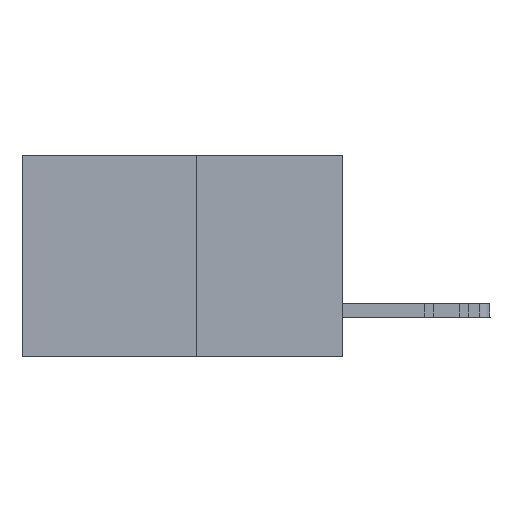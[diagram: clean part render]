
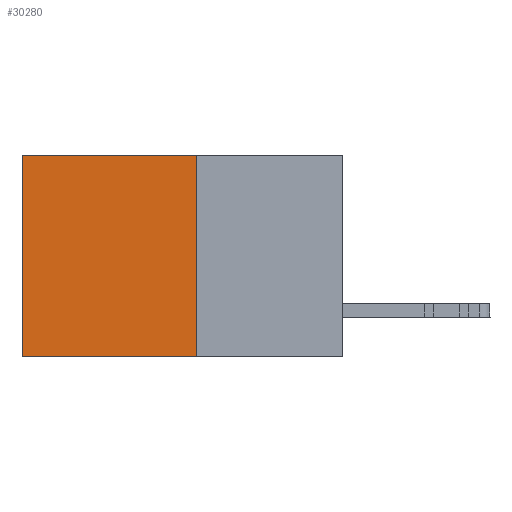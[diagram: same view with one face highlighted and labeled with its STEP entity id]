
A CAD part, left-side view. The second image highlights one B-rep face of the part: STEP entity #30280.
In plain terms, the highlighted planar face has unit normal (-1, 0, 0).
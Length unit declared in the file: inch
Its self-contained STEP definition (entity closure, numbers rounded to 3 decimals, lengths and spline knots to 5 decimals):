
#276 = VERTEX_POINT ( 'NONE', #27591 ) ;
#533 = LINE ( 'NONE', #15599, #6340 ) ;
#884 = ORIENTED_EDGE ( 'NONE', *, *, #6811, .T. ) ;
#2942 = FACE_OUTER_BOUND ( 'NONE', #16641, .T. ) ;
#3382 = DIRECTION ( 'NONE',  ( 0., 0., -1. ) ) ;
#3504 = ORIENTED_EDGE ( 'NONE', *, *, #21142, .T. ) ;
#3750 = LINE ( 'NONE', #5084, #10233 ) ;
#4756 = VERTEX_POINT ( 'NONE', #24089 ) ;
#5084 = CARTESIAN_POINT ( 'NONE',  ( 0.277, 0.27, -0.37 ) ) ;
#6340 = VECTOR ( 'NONE', #3382, 39.37008 ) ;
#6811 = EDGE_CURVE ( 'NONE', #13426, #9421, #27106, .T. ) ;
#7402 = PLANE ( 'NONE',  #9200 ) ;
#7548 = DIRECTION ( 'NONE',  ( 0., 1., 0. ) ) ;
#9200 = AXIS2_PLACEMENT_3D ( 'NONE', #23743, #9836, #27063 ) ;
#9295 = DIRECTION ( 'NONE',  ( 0., 0., -1. ) ) ;
#9328 = CARTESIAN_POINT ( 'NONE',  ( 0.277, 0.59, -0.37 ) ) ;
#9421 = VERTEX_POINT ( 'NONE', #14662 ) ;
#9836 = DIRECTION ( 'NONE',  ( 1., 0., 0. ) ) ;
#10233 = VECTOR ( 'NONE', #7548, 39.37008 ) ;
#13426 = VERTEX_POINT ( 'NONE', #31070 ) ;
#14662 = CARTESIAN_POINT ( 'NONE',  ( 0.277, 0.59, -0.37 ) ) ;
#15395 = VECTOR ( 'NONE', #19144, 39.37008 ) ;
#15599 = CARTESIAN_POINT ( 'NONE',  ( 0.277, 0.27, -0.37 ) ) ;
#16641 = EDGE_LOOP ( 'NONE', ( #884, #31341, #17680, #3504 ) ) ;
#17680 = ORIENTED_EDGE ( 'NONE', *, *, #31157, .F. ) ;
#19144 = DIRECTION ( 'NONE',  ( 0., 1., 0. ) ) ;
#19802 = VECTOR ( 'NONE', #9295, 39.37008 ) ;
#21142 = EDGE_CURVE ( 'NONE', #276, #13426, #21977, .T. ) ;
#21977 = LINE ( 'NONE', #23764, #15395 ) ;
#23743 = CARTESIAN_POINT ( 'NONE',  ( 0.277, 0.27, -0.37 ) ) ;
#23764 = CARTESIAN_POINT ( 'NONE',  ( 0.277, 0.27, 0. ) ) ;
#24089 = CARTESIAN_POINT ( 'NONE',  ( 0.277, 0.27, -0.37 ) ) ;
#27063 = DIRECTION ( 'NONE',  ( 0., 0., -1. ) ) ;
#27106 = LINE ( 'NONE', #9328, #19802 ) ;
#27591 = CARTESIAN_POINT ( 'NONE',  ( 0.277, 0.27, 0. ) ) ;
#29181 = EDGE_CURVE ( 'NONE', #4756, #9421, #3750, .T. ) ;
#30280 = ADVANCED_FACE ( 'NONE', ( #2942 ), #7402, .F. ) ;
#31070 = CARTESIAN_POINT ( 'NONE',  ( 0.277, 0.59, 0. ) ) ;
#31157 = EDGE_CURVE ( 'NONE', #276, #4756, #533, .T. ) ;
#31341 = ORIENTED_EDGE ( 'NONE', *, *, #29181, .F. ) ;
